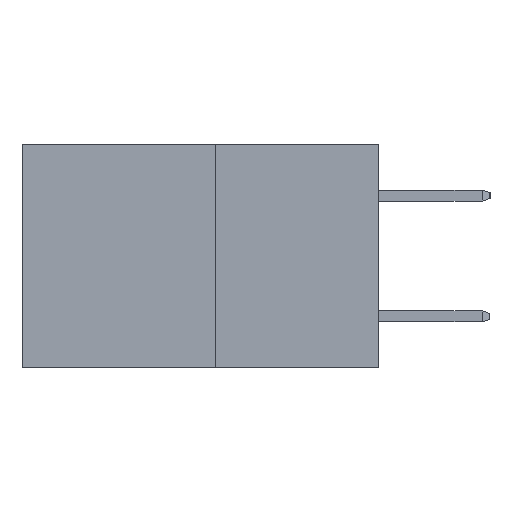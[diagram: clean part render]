
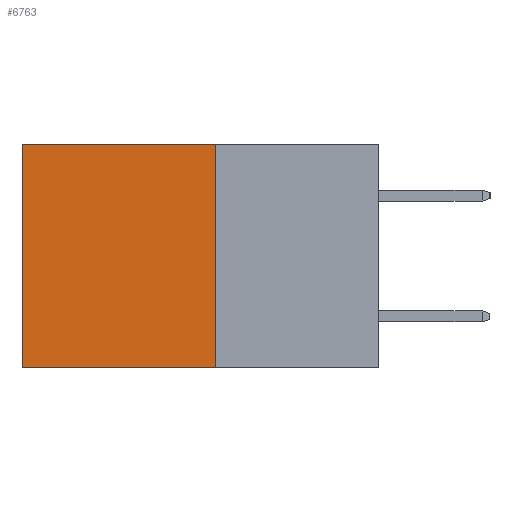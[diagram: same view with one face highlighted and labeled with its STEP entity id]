
A CAD part, left-side view. The second image highlights one B-rep face of the part: STEP entity #6763.
In plain terms, the highlighted planar face has unit normal (-1, 0, 0).
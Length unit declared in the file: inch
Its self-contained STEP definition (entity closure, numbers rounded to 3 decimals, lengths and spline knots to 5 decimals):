
#738 = CARTESIAN_POINT ( 'NONE',  ( 0.277, 0.59, -0.37 ) ) ;
#827 = VECTOR ( 'NONE', #14126, 39.37008 ) ;
#853 = VECTOR ( 'NONE', #11262, 39.37008 ) ;
#933 = CARTESIAN_POINT ( 'NONE',  ( 0.277, 0.59, -0.37 ) ) ;
#1456 = VERTEX_POINT ( 'NONE', #1830 ) ;
#1514 = CARTESIAN_POINT ( 'NONE',  ( 0.277, 0.27, -0.37 ) ) ;
#1820 = VERTEX_POINT ( 'NONE', #1514 ) ;
#1830 = CARTESIAN_POINT ( 'NONE',  ( 0.277, 0.59, 0. ) ) ;
#1921 = VECTOR ( 'NONE', #4943, 39.37008 ) ;
#1959 = VECTOR ( 'NONE', #2055, 39.37008 ) ;
#2055 = DIRECTION ( 'NONE',  ( 0., 0., -1. ) ) ;
#2359 = LINE ( 'NONE', #11436, #1959 ) ;
#2543 = CARTESIAN_POINT ( 'NONE',  ( 0.277, 0.27, 0. ) ) ;
#3411 = FACE_OUTER_BOUND ( 'NONE', #3477, .T. ) ;
#3477 = EDGE_LOOP ( 'NONE', ( #4440, #5098, #5170, #5250 ) ) ;
#4206 = LINE ( 'NONE', #738, #853 ) ;
#4216 = EDGE_CURVE ( 'NONE', #15141, #1456, #8291, .T. ) ;
#4440 = ORIENTED_EDGE ( 'NONE', *, *, #4884, .T. ) ;
#4884 = EDGE_CURVE ( 'NONE', #1456, #6559, #4206, .T. ) ;
#4943 = DIRECTION ( 'NONE',  ( 0., 1., 0. ) ) ;
#5098 = ORIENTED_EDGE ( 'NONE', *, *, #6728, .F. ) ;
#5170 = ORIENTED_EDGE ( 'NONE', *, *, #12365, .F. ) ;
#5250 = ORIENTED_EDGE ( 'NONE', *, *, #4216, .T. ) ;
#6559 = VERTEX_POINT ( 'NONE', #933 ) ;
#6728 = EDGE_CURVE ( 'NONE', #1820, #6559, #10354, .T. ) ;
#6763 = ADVANCED_FACE ( 'NONE', ( #3411 ), #13658, .F. ) ;
#8291 = LINE ( 'NONE', #11419, #1921 ) ;
#10354 = LINE ( 'NONE', #14297, #827 ) ;
#11262 = DIRECTION ( 'NONE',  ( 0., 0., -1. ) ) ;
#11419 = CARTESIAN_POINT ( 'NONE',  ( 0.277, 0.27, 0. ) ) ;
#11436 = CARTESIAN_POINT ( 'NONE',  ( 0.277, 0.27, -0.37 ) ) ;
#12365 = EDGE_CURVE ( 'NONE', #15141, #1820, #2359, .T. ) ;
#12545 = AXIS2_PLACEMENT_3D ( 'NONE', #13770, #13642, #13608 ) ;
#13608 = DIRECTION ( 'NONE',  ( 0., 0., -1. ) ) ;
#13642 = DIRECTION ( 'NONE',  ( 1., 0., 0. ) ) ;
#13658 = PLANE ( 'NONE',  #12545 ) ;
#13770 = CARTESIAN_POINT ( 'NONE',  ( 0.277, 0.27, -0.37 ) ) ;
#14126 = DIRECTION ( 'NONE',  ( 0., 1., 0. ) ) ;
#14297 = CARTESIAN_POINT ( 'NONE',  ( 0.277, 0.27, -0.37 ) ) ;
#15141 = VERTEX_POINT ( 'NONE', #2543 ) ;
